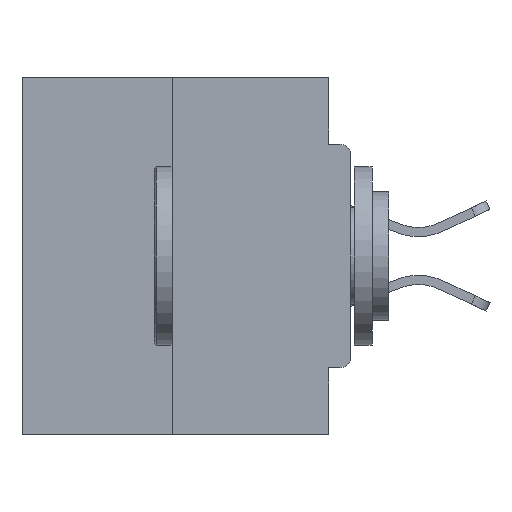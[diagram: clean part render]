
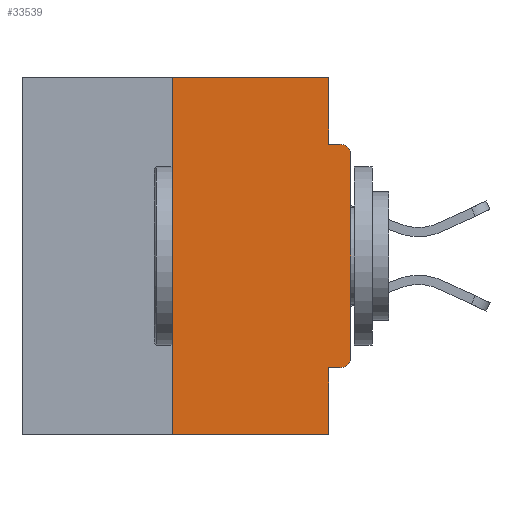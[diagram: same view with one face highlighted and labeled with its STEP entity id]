
A CAD part, left-side view. The second image highlights one B-rep face of the part: STEP entity #33539.
In plain terms, the highlighted planar face has unit normal (-1, 0, 0).
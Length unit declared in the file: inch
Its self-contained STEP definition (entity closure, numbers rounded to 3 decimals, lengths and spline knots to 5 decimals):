
#176 = CARTESIAN_POINT ( 'NONE',  ( 0., 0.25, 0. ) ) ;
#774 = VERTEX_POINT ( 'NONE', #6944 ) ;
#937 = EDGE_CURVE ( 'NONE', #7824, #15499, #7642, .T. ) ;
#1138 = CARTESIAN_POINT ( 'NONE',  ( 0., 0.46, 0. ) ) ;
#1149 = EDGE_CURVE ( 'NONE', #11239, #7824, #12651, .T. ) ;
#1853 = DIRECTION ( 'NONE',  ( 0., 0., -1. ) ) ;
#2119 = DIRECTION ( 'NONE',  ( 0., -1., 0. ) ) ;
#2214 = DIRECTION ( 'NONE',  ( 0., 0., 1. ) ) ;
#2356 = ORIENTED_EDGE ( 'NONE', *, *, #1149, .F. ) ;
#2425 = CARTESIAN_POINT ( 'NONE',  ( 0., 0.031, -0.0935 ) ) ;
#3409 = LINE ( 'NONE', #22251, #7226 ) ;
#3468 = CARTESIAN_POINT ( 'NONE',  ( 0., 0.25, -0.5 ) ) ;
#4240 = PLANE ( 'NONE',  #15659 ) ;
#4275 = AXIS2_PLACEMENT_3D ( 'NONE', #20018, #17979, #1853 ) ;
#4432 = DIRECTION ( 'NONE',  ( 0., 0., -1. ) ) ;
#5026 = CARTESIAN_POINT ( 'NONE',  ( 0., 0.031, -0.5 ) ) ;
#6944 = CARTESIAN_POINT ( 'NONE',  ( 0., 0., -0.3915 ) ) ;
#7226 = VECTOR ( 'NONE', #8709, 39.37008 ) ;
#7631 = DIRECTION ( 'NONE',  ( 0., 0., -1. ) ) ;
#7642 = LINE ( 'NONE', #5026, #34042 ) ;
#7824 = VERTEX_POINT ( 'NONE', #20613 ) ;
#8709 = DIRECTION ( 'NONE',  ( 0., -1., 0. ) ) ;
#8983 = VERTEX_POINT ( 'NONE', #31841 ) ;
#8992 = ORIENTED_EDGE ( 'NONE', *, *, #32863, .T. ) ;
#9208 = EDGE_LOOP ( 'NONE', ( #9605, #20531, #8992, #33514, #2356, #14195, #30743, #10925, #20681, #9739 ) ) ;
#9605 = ORIENTED_EDGE ( 'NONE', *, *, #32582, .F. ) ;
#9739 = ORIENTED_EDGE ( 'NONE', *, *, #31281, .F. ) ;
#9839 = CARTESIAN_POINT ( 'NONE',  ( 0., 0.46, 0. ) ) ;
#10077 = CARTESIAN_POINT ( 'NONE',  ( 0., 0.46, -0.5 ) ) ;
#10138 = CARTESIAN_POINT ( 'NONE',  ( 0., 0.25, 0. ) ) ;
#10411 = DIRECTION ( 'NONE',  ( 0., -1., 0. ) ) ;
#10655 = LINE ( 'NONE', #10138, #34999 ) ;
#10925 = ORIENTED_EDGE ( 'NONE', *, *, #27835, .T. ) ;
#11239 = VERTEX_POINT ( 'NONE', #26785 ) ;
#11397 = LINE ( 'NONE', #10077, #14357 ) ;
#12491 = CARTESIAN_POINT ( 'NONE',  ( 0., 0.015, -0.0935 ) ) ;
#12651 = LINE ( 'NONE', #18810, #31415 ) ;
#13979 = VERTEX_POINT ( 'NONE', #32349 ) ;
#14195 = ORIENTED_EDGE ( 'NONE', *, *, #17331, .T. ) ;
#14357 = VECTOR ( 'NONE', #10411, 39.37008 ) ;
#15106 = EDGE_CURVE ( 'NONE', #30560, #17411, #3409, .T. ) ;
#15499 = VERTEX_POINT ( 'NONE', #34937 ) ;
#15659 = AXIS2_PLACEMENT_3D ( 'NONE', #1138, #28219, #20147 ) ;
#17331 = EDGE_CURVE ( 'NONE', #11239, #774, #29528, .T. ) ;
#17411 = VERTEX_POINT ( 'NONE', #12491 ) ;
#17684 = VERTEX_POINT ( 'NONE', #176 ) ;
#17979 = DIRECTION ( 'NONE',  ( -1., 0., 0. ) ) ;
#18810 = CARTESIAN_POINT ( 'NONE',  ( 0., 0., -0.4065 ) ) ;
#19462 = EDGE_CURVE ( 'NONE', #774, #13979, #20463, .T. ) ;
#19836 = DIRECTION ( 'NONE',  ( 0., 0., 1. ) ) ;
#20018 = CARTESIAN_POINT ( 'NONE',  ( 0., 0.015, -0.3915 ) ) ;
#20147 = DIRECTION ( 'NONE',  ( 0., 0., -1. ) ) ;
#20463 = LINE ( 'NONE', #33049, #25996 ) ;
#20531 = ORIENTED_EDGE ( 'NONE', *, *, #26441, .F. ) ;
#20613 = CARTESIAN_POINT ( 'NONE',  ( 0., 0.031, -0.4065 ) ) ;
#20681 = ORIENTED_EDGE ( 'NONE', *, *, #15106, .F. ) ;
#22251 = CARTESIAN_POINT ( 'NONE',  ( 0., 0., -0.0935 ) ) ;
#22425 = DIRECTION ( 'NONE',  ( 0., 0., -1. ) ) ;
#22675 = AXIS2_PLACEMENT_3D ( 'NONE', #35224, #26146, #4432 ) ;
#25049 = CIRCLE ( 'NONE', #22675, 0.015 ) ;
#25996 = VECTOR ( 'NONE', #19836, 39.37008 ) ;
#26146 = DIRECTION ( 'NONE',  ( -1., 0., 0. ) ) ;
#26441 = EDGE_CURVE ( 'NONE', #26972, #17684, #10655, .T. ) ;
#26785 = CARTESIAN_POINT ( 'NONE',  ( 0., 0.015, -0.4065 ) ) ;
#26888 = DIRECTION ( 'NONE',  ( 0., 1., 0. ) ) ;
#26972 = VERTEX_POINT ( 'NONE', #3468 ) ;
#27659 = LINE ( 'NONE', #27669, #31482 ) ;
#27669 = CARTESIAN_POINT ( 'NONE',  ( 0., 0.031, 0. ) ) ;
#27835 = EDGE_CURVE ( 'NONE', #13979, #17411, #25049, .T. ) ;
#28219 = DIRECTION ( 'NONE',  ( 1., 0., 0. ) ) ;
#28438 = VECTOR ( 'NONE', #2119, 39.37008 ) ;
#29528 = CIRCLE ( 'NONE', #4275, 0.015 ) ;
#30560 = VERTEX_POINT ( 'NONE', #2425 ) ;
#30743 = ORIENTED_EDGE ( 'NONE', *, *, #19462, .T. ) ;
#31002 = LINE ( 'NONE', #9839, #28438 ) ;
#31281 = EDGE_CURVE ( 'NONE', #8983, #30560, #27659, .T. ) ;
#31415 = VECTOR ( 'NONE', #26888, 39.37008 ) ;
#31482 = VECTOR ( 'NONE', #22425, 39.37008 ) ;
#31841 = CARTESIAN_POINT ( 'NONE',  ( 0., 0.031, 0. ) ) ;
#32349 = CARTESIAN_POINT ( 'NONE',  ( 0., 0., -0.1085 ) ) ;
#32582 = EDGE_CURVE ( 'NONE', #17684, #8983, #31002, .T. ) ;
#32863 = EDGE_CURVE ( 'NONE', #26972, #15499, #11397, .T. ) ;
#33049 = CARTESIAN_POINT ( 'NONE',  ( 0., 0., 0. ) ) ;
#33514 = ORIENTED_EDGE ( 'NONE', *, *, #937, .F. ) ;
#33539 = ADVANCED_FACE ( 'NONE', ( #34357 ), #4240, .F. ) ;
#34042 = VECTOR ( 'NONE', #7631, 39.37008 ) ;
#34357 = FACE_OUTER_BOUND ( 'NONE', #9208, .T. ) ;
#34937 = CARTESIAN_POINT ( 'NONE',  ( 0., 0.031, -0.5 ) ) ;
#34999 = VECTOR ( 'NONE', #2214, 39.37008 ) ;
#35224 = CARTESIAN_POINT ( 'NONE',  ( 0., 0.015, -0.1085 ) ) ;
